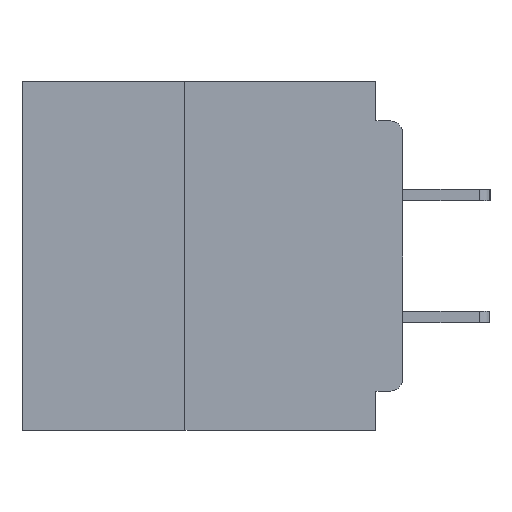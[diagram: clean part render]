
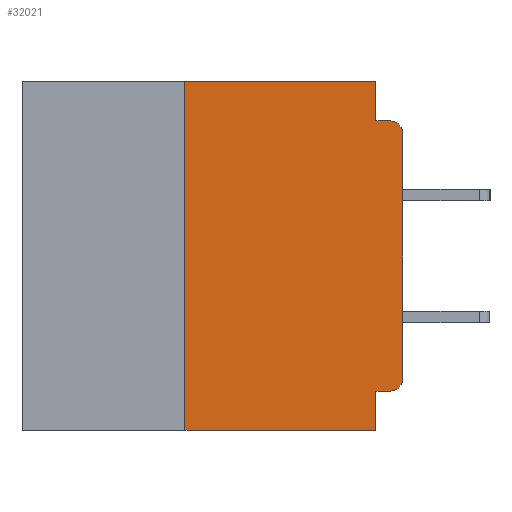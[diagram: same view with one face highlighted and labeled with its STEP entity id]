
A CAD part, left-side view. The second image highlights one B-rep face of the part: STEP entity #32021.
In plain terms, the highlighted planar face has unit normal (-1, 0, 0).
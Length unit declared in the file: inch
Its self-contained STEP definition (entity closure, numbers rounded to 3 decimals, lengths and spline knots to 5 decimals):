
#906 = AXIS2_PLACEMENT_3D ( 'NONE', #1705, #17380, #53533 ) ;
#931 = LINE ( 'NONE', #38358, #40648 ) ;
#1168 = VERTEX_POINT ( 'NONE', #45714 ) ;
#1705 = CARTESIAN_POINT ( 'NONE',  ( 0., 0.437, 0. ) ) ;
#1977 = DIRECTION ( 'NONE',  ( 0., 1., 0. ) ) ;
#2173 = EDGE_CURVE ( 'NONE', #27020, #33546, #931, .T. ) ;
#2529 = LINE ( 'NONE', #6011, #14741 ) ;
#4385 = CARTESIAN_POINT ( 'NONE',  ( 0., 0.437, 0. ) ) ;
#4699 = LINE ( 'NONE', #31947, #7985 ) ;
#4897 = AXIS2_PLACEMENT_3D ( 'NONE', #16359, #52509, #21542 ) ;
#6011 = CARTESIAN_POINT ( 'NONE',  ( 0., 0., 0. ) ) ;
#6552 = CARTESIAN_POINT ( 'NONE',  ( 0., 0.031, -0.355 ) ) ;
#7411 = VERTEX_POINT ( 'NONE', #21472 ) ;
#7985 = VECTOR ( 'NONE', #37138, 39.37008 ) ;
#8094 = LINE ( 'NONE', #60181, #34037 ) ;
#9632 = DIRECTION ( 'NONE',  ( 0., -1., 0. ) ) ;
#11247 = DIRECTION ( 'NONE',  ( 0., 0., 1. ) ) ;
#11284 = CARTESIAN_POINT ( 'NONE',  ( 0., 0.015, -0.34 ) ) ;
#12194 = PLANE ( 'NONE',  #906 ) ;
#12923 = DIRECTION ( 'NONE',  ( 0., 0., 1. ) ) ;
#13803 = CARTESIAN_POINT ( 'NONE',  ( 0., 0.031, -0.4 ) ) ;
#14741 = VECTOR ( 'NONE', #11247, 39.37008 ) ;
#15465 = AXIS2_PLACEMENT_3D ( 'NONE', #11284, #47439, #16483 ) ;
#16359 = CARTESIAN_POINT ( 'NONE',  ( 0., 0.015, -0.06 ) ) ;
#16483 = DIRECTION ( 'NONE',  ( 0., 0., -1. ) ) ;
#17052 = LINE ( 'NONE', #59194, #30816 ) ;
#17380 = DIRECTION ( 'NONE',  ( 1., 0., 0. ) ) ;
#17388 = VERTEX_POINT ( 'NONE', #54159 ) ;
#19372 = EDGE_CURVE ( 'NONE', #45022, #33546, #8094, .T. ) ;
#20862 = CIRCLE ( 'NONE', #15465, 0.015 ) ;
#21073 = ORIENTED_EDGE ( 'NONE', *, *, #64929, .T. ) ;
#21465 = LINE ( 'NONE', #22781, #61056 ) ;
#21472 = CARTESIAN_POINT ( 'NONE',  ( 0., 0.015, -0.355 ) ) ;
#21542 = DIRECTION ( 'NONE',  ( 0., 0., -1. ) ) ;
#22675 = LINE ( 'NONE', #33053, #36443 ) ;
#22781 = CARTESIAN_POINT ( 'NONE',  ( 0., 0., -0.045 ) ) ;
#23375 = ORIENTED_EDGE ( 'NONE', *, *, #59818, .F. ) ;
#25413 = ORIENTED_EDGE ( 'NONE', *, *, #43188, .T. ) ;
#25722 = ORIENTED_EDGE ( 'NONE', *, *, #50499, .F. ) ;
#26319 = VERTEX_POINT ( 'NONE', #31320 ) ;
#27020 = VERTEX_POINT ( 'NONE', #6552 ) ;
#29803 = EDGE_CURVE ( 'NONE', #7411, #27020, #22675, .T. ) ;
#30816 = VECTOR ( 'NONE', #12923, 39.37008 ) ;
#31084 = ORIENTED_EDGE ( 'NONE', *, *, #2173, .F. ) ;
#31320 = CARTESIAN_POINT ( 'NONE',  ( 0., 0., -0.34 ) ) ;
#31730 = ORIENTED_EDGE ( 'NONE', *, *, #29803, .F. ) ;
#31947 = CARTESIAN_POINT ( 'NONE',  ( 0., 0.031, 0. ) ) ;
#32021 = ADVANCED_FACE ( 'NONE', ( #42929 ), #12194, .F. ) ;
#32408 = EDGE_CURVE ( 'NONE', #17388, #57107, #33976, .T. ) ;
#32907 = CARTESIAN_POINT ( 'NONE',  ( 0., 0.031, -0.045 ) ) ;
#33053 = CARTESIAN_POINT ( 'NONE',  ( 0., 0., -0.355 ) ) ;
#33546 = VERTEX_POINT ( 'NONE', #13803 ) ;
#33976 = LINE ( 'NONE', #4385, #59782 ) ;
#34037 = VECTOR ( 'NONE', #44850, 39.37008 ) ;
#34612 = CARTESIAN_POINT ( 'NONE',  ( 0., 0.25, -0.4 ) ) ;
#36443 = VECTOR ( 'NONE', #1977, 39.37008 ) ;
#37138 = DIRECTION ( 'NONE',  ( 0., 0., -1. ) ) ;
#37445 = VERTEX_POINT ( 'NONE', #32907 ) ;
#38134 = DIRECTION ( 'NONE',  ( 0., 0., -1. ) ) ;
#38358 = CARTESIAN_POINT ( 'NONE',  ( 0., 0.031, -0.4 ) ) ;
#39780 = EDGE_CURVE ( 'NONE', #57107, #37445, #4699, .T. ) ;
#40648 = VECTOR ( 'NONE', #38134, 39.37008 ) ;
#42242 = ORIENTED_EDGE ( 'NONE', *, *, #39780, .F. ) ;
#42929 = FACE_OUTER_BOUND ( 'NONE', #64657, .T. ) ;
#43188 = EDGE_CURVE ( 'NONE', #1168, #53252, #53264, .T. ) ;
#44850 = DIRECTION ( 'NONE',  ( 0., -1., 0. ) ) ;
#45022 = VERTEX_POINT ( 'NONE', #34612 ) ;
#45714 = CARTESIAN_POINT ( 'NONE',  ( 0., 0., -0.06 ) ) ;
#47439 = DIRECTION ( 'NONE',  ( -1., 0., 0. ) ) ;
#48777 = DIRECTION ( 'NONE',  ( 0., -1., 0. ) ) ;
#50499 = EDGE_CURVE ( 'NONE', #37445, #53252, #21465, .T. ) ;
#52509 = DIRECTION ( 'NONE',  ( -1., 0., 0. ) ) ;
#53252 = VERTEX_POINT ( 'NONE', #57597 ) ;
#53264 = CIRCLE ( 'NONE', #4897, 0.015 ) ;
#53533 = DIRECTION ( 'NONE',  ( 0., 0., -1. ) ) ;
#54159 = CARTESIAN_POINT ( 'NONE',  ( 0., 0.25, 0. ) ) ;
#56792 = ORIENTED_EDGE ( 'NONE', *, *, #19372, .T. ) ;
#57107 = VERTEX_POINT ( 'NONE', #66160 ) ;
#57597 = CARTESIAN_POINT ( 'NONE',  ( 0., 0.015, -0.045 ) ) ;
#59194 = CARTESIAN_POINT ( 'NONE',  ( 0., 0.25, -0.4 ) ) ;
#59782 = VECTOR ( 'NONE', #9632, 39.37008 ) ;
#59818 = EDGE_CURVE ( 'NONE', #45022, #17388, #17052, .T. ) ;
#60181 = CARTESIAN_POINT ( 'NONE',  ( 0., 0.437, -0.4 ) ) ;
#61056 = VECTOR ( 'NONE', #48777, 39.37008 ) ;
#61683 = ORIENTED_EDGE ( 'NONE', *, *, #32408, .F. ) ;
#63632 = ORIENTED_EDGE ( 'NONE', *, *, #66999, .T. ) ;
#64657 = EDGE_LOOP ( 'NONE', ( #63632, #25413, #25722, #42242, #61683, #23375, #56792, #31084, #31730, #21073 ) ) ;
#64929 = EDGE_CURVE ( 'NONE', #7411, #26319, #20862, .T. ) ;
#66160 = CARTESIAN_POINT ( 'NONE',  ( 0., 0.031, 0. ) ) ;
#66999 = EDGE_CURVE ( 'NONE', #26319, #1168, #2529, .T. ) ;
